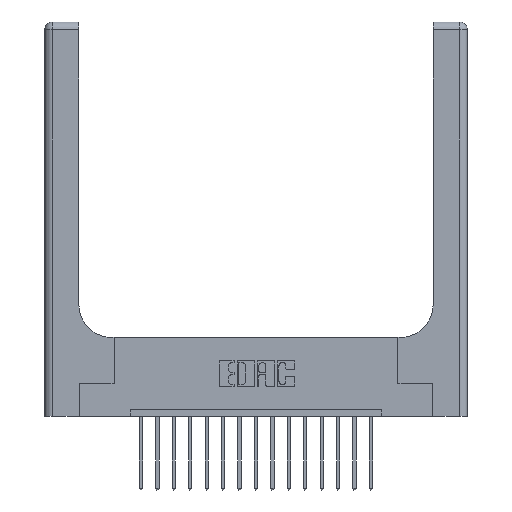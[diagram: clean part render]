
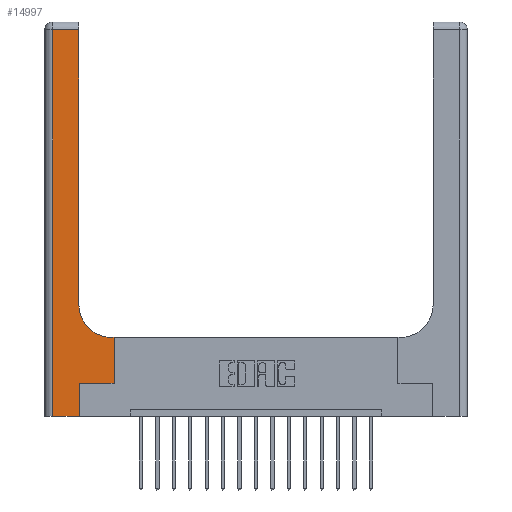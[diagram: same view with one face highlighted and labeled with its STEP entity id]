
A CAD part, top view. The second image highlights one B-rep face of the part: STEP entity #14997.
In plain terms, the highlighted planar face has unit normal (0, 0, 1).
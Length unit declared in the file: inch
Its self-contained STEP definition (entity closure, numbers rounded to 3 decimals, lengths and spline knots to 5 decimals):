
#185 = DIRECTION ( 'NONE',  ( 0., 0., -1. ) ) ;
#476 = FACE_OUTER_BOUND ( 'NONE', #6094, .T. ) ;
#1133 = VERTEX_POINT ( 'NONE', #1396 ) ;
#1396 = CARTESIAN_POINT ( 'NONE',  ( 0.528, 0.25, 0.37 ) ) ;
#1402 = VERTEX_POINT ( 'NONE', #15538 ) ;
#1443 = ORIENTED_EDGE ( 'NONE', *, *, #4462, .T. ) ;
#1790 = CARTESIAN_POINT ( 'NONE',  ( 0., 3., 0.37 ) ) ;
#1886 = PLANE ( 'NONE',  #6813 ) ;
#2109 = EDGE_CURVE ( 'NONE', #9383, #5337, #16069, .T. ) ;
#2327 = CARTESIAN_POINT ( 'NONE',  ( 0.265, 0.25, 0.37 ) ) ;
#2392 = LINE ( 'NONE', #5396, #13492 ) ;
#2703 = ORIENTED_EDGE ( 'NONE', *, *, #10340, .T. ) ;
#3716 = CARTESIAN_POINT ( 'NONE',  ( 0.26, 0.85, 0.37 ) ) ;
#3734 = LINE ( 'NONE', #2327, #10015 ) ;
#3827 = DIRECTION ( 'NONE',  ( 1., 0., 0. ) ) ;
#3876 = VECTOR ( 'NONE', #12284, 39.37008 ) ;
#4255 = VERTEX_POINT ( 'NONE', #4926 ) ;
#4316 = CARTESIAN_POINT ( 'NONE',  ( 0.528, 0.6, 0.37 ) ) ;
#4416 = CARTESIAN_POINT ( 'NONE',  ( 0.51, 0.85, 0.37 ) ) ;
#4462 = EDGE_CURVE ( 'NONE', #10513, #1402, #9586, .T. ) ;
#4659 = ORIENTED_EDGE ( 'NONE', *, *, #2109, .T. ) ;
#4855 = EDGE_CURVE ( 'NONE', #1402, #13356, #18052, .T. ) ;
#4926 = CARTESIAN_POINT ( 'NONE',  ( 0.26, 2.94, 0.37 ) ) ;
#5155 = DIRECTION ( 'NONE',  ( 0., 1., 0. ) ) ;
#5302 = DIRECTION ( 'NONE',  ( -1., 0., 0. ) ) ;
#5337 = VERTEX_POINT ( 'NONE', #3716 ) ;
#5396 = CARTESIAN_POINT ( 'NONE',  ( 0.06, 3., 0.37 ) ) ;
#5823 = VERTEX_POINT ( 'NONE', #16959 ) ;
#6094 = EDGE_LOOP ( 'NONE', ( #6431, #12325, #16684, #1443, #8231, #6695, #2703, #9792, #4659 ) ) ;
#6431 = ORIENTED_EDGE ( 'NONE', *, *, #12691, .T. ) ;
#6653 = CARTESIAN_POINT ( 'NONE',  ( 0.265, 0., 0.37 ) ) ;
#6695 = ORIENTED_EDGE ( 'NONE', *, *, #10555, .T. ) ;
#6813 = AXIS2_PLACEMENT_3D ( 'NONE', #1790, #185, #11749 ) ;
#6851 = CARTESIAN_POINT ( 'NONE',  ( 0., 0., 0.37 ) ) ;
#6973 = CARTESIAN_POINT ( 'NONE',  ( 0., 2.94, 0.37 ) ) ;
#7220 = DIRECTION ( 'NONE',  ( 1., 0., 0. ) ) ;
#7980 = VECTOR ( 'NONE', #5155, 39.37008 ) ;
#8196 = LINE ( 'NONE', #9884, #18057 ) ;
#8231 = ORIENTED_EDGE ( 'NONE', *, *, #4855, .T. ) ;
#8300 = DIRECTION ( 'NONE',  ( 0., -1., 0. ) ) ;
#8378 = VECTOR ( 'NONE', #5302, 39.37008 ) ;
#8574 = LINE ( 'NONE', #6973, #8378 ) ;
#8907 = DIRECTION ( 'NONE',  ( 0., 1., 0. ) ) ;
#9193 = CARTESIAN_POINT ( 'NONE',  ( 0.06, 0., 0.37 ) ) ;
#9383 = VERTEX_POINT ( 'NONE', #14531 ) ;
#9586 = LINE ( 'NONE', #6851, #14554 ) ;
#9746 = AXIS2_PLACEMENT_3D ( 'NONE', #4416, #10232, #7220 ) ;
#9792 = ORIENTED_EDGE ( 'NONE', *, *, #13459, .T. ) ;
#9884 = CARTESIAN_POINT ( 'NONE',  ( 0.26, 3., 0.37 ) ) ;
#10015 = VECTOR ( 'NONE', #3827, 39.37008 ) ;
#10232 = DIRECTION ( 'NONE',  ( 0., 0., -1. ) ) ;
#10340 = EDGE_CURVE ( 'NONE', #1133, #18425, #15974, .T. ) ;
#10513 = VERTEX_POINT ( 'NONE', #9193 ) ;
#10555 = EDGE_CURVE ( 'NONE', #13356, #1133, #3734, .T. ) ;
#11007 = DIRECTION ( 'NONE',  ( 1., 0., 0. ) ) ;
#11749 = DIRECTION ( 'NONE',  ( -1., 0., 0. ) ) ;
#12284 = DIRECTION ( 'NONE',  ( -1., 0., 0. ) ) ;
#12325 = ORIENTED_EDGE ( 'NONE', *, *, #16949, .T. ) ;
#12691 = EDGE_CURVE ( 'NONE', #5337, #4255, #8196, .T. ) ;
#13356 = VERTEX_POINT ( 'NONE', #17848 ) ;
#13459 = EDGE_CURVE ( 'NONE', #18425, #9383, #13782, .T. ) ;
#13492 = VECTOR ( 'NONE', #8300, 39.37008 ) ;
#13782 = LINE ( 'NONE', #13871, #3876 ) ;
#13871 = CARTESIAN_POINT ( 'NONE',  ( 0.26, 0.6, 0.37 ) ) ;
#14511 = VECTOR ( 'NONE', #8907, 39.37008 ) ;
#14531 = CARTESIAN_POINT ( 'NONE',  ( 0.51, 0.6, 0.37 ) ) ;
#14554 = VECTOR ( 'NONE', #11007, 39.37008 ) ;
#14641 = CARTESIAN_POINT ( 'NONE',  ( 0.528, 0.25, 0.37 ) ) ;
#14997 = ADVANCED_FACE ( 'NONE', ( #476 ), #1886, .F. ) ;
#15538 = CARTESIAN_POINT ( 'NONE',  ( 0.265, 0., 0.37 ) ) ;
#15974 = LINE ( 'NONE', #14641, #14511 ) ;
#16069 = CIRCLE ( 'NONE', #9746, 0.25 ) ;
#16684 = ORIENTED_EDGE ( 'NONE', *, *, #16948, .T. ) ;
#16948 = EDGE_CURVE ( 'NONE', #5823, #10513, #2392, .T. ) ;
#16949 = EDGE_CURVE ( 'NONE', #4255, #5823, #8574, .T. ) ;
#16959 = CARTESIAN_POINT ( 'NONE',  ( 0.06, 2.94, 0.37 ) ) ;
#17848 = CARTESIAN_POINT ( 'NONE',  ( 0.265, 0.25, 0.37 ) ) ;
#18052 = LINE ( 'NONE', #6653, #7980 ) ;
#18057 = VECTOR ( 'NONE', #18376, 39.37008 ) ;
#18376 = DIRECTION ( 'NONE',  ( 0., 1., 0. ) ) ;
#18425 = VERTEX_POINT ( 'NONE', #4316 ) ;
